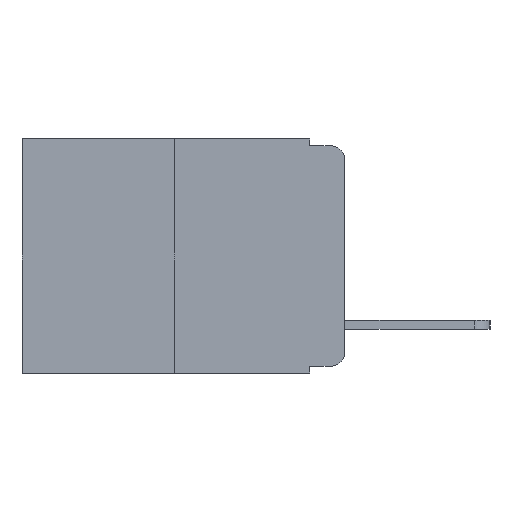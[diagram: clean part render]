
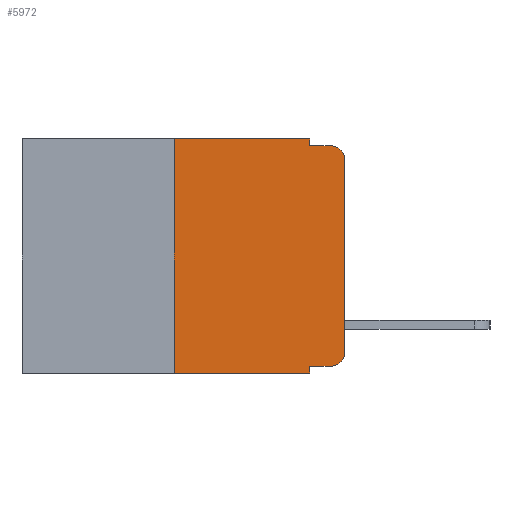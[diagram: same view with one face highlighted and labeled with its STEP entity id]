
A CAD part, left-side view. The second image highlights one B-rep face of the part: STEP entity #5972.
In plain terms, the highlighted planar face has unit normal (-1, 0, 0).
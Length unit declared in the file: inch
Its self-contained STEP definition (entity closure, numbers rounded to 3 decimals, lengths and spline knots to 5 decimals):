
#143 = CARTESIAN_POINT ( 'NONE',  ( 0., 0.051, -0.01 ) ) ;
#603 = AXIS2_PLACEMENT_3D ( 'NONE', #6913, #15549, #4208 ) ;
#701 = ORIENTED_EDGE ( 'NONE', *, *, #5323, .T. ) ;
#977 = DIRECTION ( 'NONE',  ( 0., 0., -1. ) ) ;
#1059 = DIRECTION ( 'NONE',  ( 0., 0., 1. ) ) ;
#1159 = DIRECTION ( 'NONE',  ( 0., 0., -1. ) ) ;
#1422 = LINE ( 'NONE', #2627, #9577 ) ;
#1492 = VECTOR ( 'NONE', #1059, 39.37008 ) ;
#1866 = VERTEX_POINT ( 'NONE', #9446 ) ;
#2014 = EDGE_CURVE ( 'NONE', #9485, #1866, #4151, .T. ) ;
#2132 = CARTESIAN_POINT ( 'NONE',  ( 0., 0.02, -0.333 ) ) ;
#2362 = CARTESIAN_POINT ( 'NONE',  ( 0., 0.473, 0. ) ) ;
#2540 = CARTESIAN_POINT ( 'NONE',  ( 0., 0., -0.03 ) ) ;
#2627 = CARTESIAN_POINT ( 'NONE',  ( 0., 0.051, 0. ) ) ;
#2726 = AXIS2_PLACEMENT_3D ( 'NONE', #6661, #8140, #1159 ) ;
#3242 = VECTOR ( 'NONE', #7519, 39.37008 ) ;
#3527 = DIRECTION ( 'NONE',  ( 0., -1., 0. ) ) ;
#3655 = EDGE_CURVE ( 'NONE', #11890, #4859, #13785, .T. ) ;
#3767 = FACE_OUTER_BOUND ( 'NONE', #18358, .T. ) ;
#4101 = ORIENTED_EDGE ( 'NONE', *, *, #14394, .F. ) ;
#4151 = LINE ( 'NONE', #5627, #9805 ) ;
#4208 = DIRECTION ( 'NONE',  ( 0., 0., -1. ) ) ;
#4634 = LINE ( 'NONE', #17569, #7781 ) ;
#4705 = VERTEX_POINT ( 'NONE', #9137 ) ;
#4762 = EDGE_CURVE ( 'NONE', #12886, #11890, #14232, .T. ) ;
#4859 = VERTEX_POINT ( 'NONE', #2540 ) ;
#5000 = ORIENTED_EDGE ( 'NONE', *, *, #18003, .T. ) ;
#5323 = EDGE_CURVE ( 'NONE', #12598, #12886, #11717, .T. ) ;
#5627 = CARTESIAN_POINT ( 'NONE',  ( 0., 0.051, -0.01 ) ) ;
#5905 = DIRECTION ( 'NONE',  ( 0., -1., 0. ) ) ;
#5927 = VERTEX_POINT ( 'NONE', #8210 ) ;
#5972 = ADVANCED_FACE ( 'NONE', ( #3767 ), #9421, .F. ) ;
#6021 = EDGE_CURVE ( 'NONE', #12598, #4705, #1422, .T. ) ;
#6317 = VERTEX_POINT ( 'NONE', #16400 ) ;
#6661 = CARTESIAN_POINT ( 'NONE',  ( 0., 0.02, -0.03 ) ) ;
#6913 = CARTESIAN_POINT ( 'NONE',  ( 0., 0.02, -0.313 ) ) ;
#7011 = CARTESIAN_POINT ( 'NONE',  ( 0., 0.051, 0. ) ) ;
#7519 = DIRECTION ( 'NONE',  ( 0., -1., 0. ) ) ;
#7607 = DIRECTION ( 'NONE',  ( 0., 0., 1. ) ) ;
#7736 = VECTOR ( 'NONE', #7607, 39.37008 ) ;
#7781 = VECTOR ( 'NONE', #3527, 39.37008 ) ;
#7793 = AXIS2_PLACEMENT_3D ( 'NONE', #2362, #8031, #977 ) ;
#8031 = DIRECTION ( 'NONE',  ( 1., 0., 0. ) ) ;
#8140 = DIRECTION ( 'NONE',  ( -1., 0., 0. ) ) ;
#8210 = CARTESIAN_POINT ( 'NONE',  ( 0., 0.25, 0. ) ) ;
#8428 = ORIENTED_EDGE ( 'NONE', *, *, #12891, .T. ) ;
#9137 = CARTESIAN_POINT ( 'NONE',  ( 0., 0.051, -0.343 ) ) ;
#9271 = CIRCLE ( 'NONE', #2726, 0.02 ) ;
#9421 = PLANE ( 'NONE',  #7793 ) ;
#9430 = EDGE_CURVE ( 'NONE', #6317, #9485, #14065, .T. ) ;
#9446 = CARTESIAN_POINT ( 'NONE',  ( 0., 0.02, -0.01 ) ) ;
#9485 = VERTEX_POINT ( 'NONE', #143 ) ;
#9540 = ORIENTED_EDGE ( 'NONE', *, *, #9430, .F. ) ;
#9577 = VECTOR ( 'NONE', #14064, 39.37008 ) ;
#9805 = VECTOR ( 'NONE', #18009, 39.37008 ) ;
#10108 = CARTESIAN_POINT ( 'NONE',  ( 0., 0.473, 0. ) ) ;
#10598 = ORIENTED_EDGE ( 'NONE', *, *, #6021, .F. ) ;
#11717 = LINE ( 'NONE', #17392, #3242 ) ;
#11789 = LINE ( 'NONE', #14758, #7736 ) ;
#11890 = VERTEX_POINT ( 'NONE', #12604 ) ;
#12586 = CARTESIAN_POINT ( 'NONE',  ( 0., 0., 0. ) ) ;
#12598 = VERTEX_POINT ( 'NONE', #12650 ) ;
#12604 = CARTESIAN_POINT ( 'NONE',  ( 0., 0., -0.313 ) ) ;
#12631 = VECTOR ( 'NONE', #12686, 39.37008 ) ;
#12650 = CARTESIAN_POINT ( 'NONE',  ( 0., 0.051, -0.333 ) ) ;
#12686 = DIRECTION ( 'NONE',  ( 0., 0., -1. ) ) ;
#12886 = VERTEX_POINT ( 'NONE', #2132 ) ;
#12891 = EDGE_CURVE ( 'NONE', #13789, #4705, #4634, .T. ) ;
#12948 = ORIENTED_EDGE ( 'NONE', *, *, #16111, .F. ) ;
#13671 = CARTESIAN_POINT ( 'NONE',  ( 0., 0.25, -0.343 ) ) ;
#13785 = LINE ( 'NONE', #12586, #1492 ) ;
#13789 = VERTEX_POINT ( 'NONE', #13671 ) ;
#14064 = DIRECTION ( 'NONE',  ( 0., 0., -1. ) ) ;
#14065 = LINE ( 'NONE', #7011, #12631 ) ;
#14182 = LINE ( 'NONE', #10108, #14479 ) ;
#14232 = CIRCLE ( 'NONE', #603, 0.02 ) ;
#14394 = EDGE_CURVE ( 'NONE', #5927, #6317, #14182, .T. ) ;
#14423 = ORIENTED_EDGE ( 'NONE', *, *, #4762, .T. ) ;
#14479 = VECTOR ( 'NONE', #5905, 39.37008 ) ;
#14758 = CARTESIAN_POINT ( 'NONE',  ( 0., 0.25, 0. ) ) ;
#15426 = ORIENTED_EDGE ( 'NONE', *, *, #3655, .T. ) ;
#15549 = DIRECTION ( 'NONE',  ( -1., 0., 0. ) ) ;
#15809 = ORIENTED_EDGE ( 'NONE', *, *, #2014, .F. ) ;
#16111 = EDGE_CURVE ( 'NONE', #13789, #5927, #11789, .T. ) ;
#16400 = CARTESIAN_POINT ( 'NONE',  ( 0., 0.051, 0. ) ) ;
#17392 = CARTESIAN_POINT ( 'NONE',  ( 0., 0.051, -0.333 ) ) ;
#17569 = CARTESIAN_POINT ( 'NONE',  ( 0., 0.473, -0.343 ) ) ;
#18003 = EDGE_CURVE ( 'NONE', #4859, #1866, #9271, .T. ) ;
#18009 = DIRECTION ( 'NONE',  ( 0., -1., 0. ) ) ;
#18358 = EDGE_LOOP ( 'NONE', ( #15426, #5000, #15809, #9540, #4101, #12948, #8428, #10598, #701, #14423 ) ) ;
